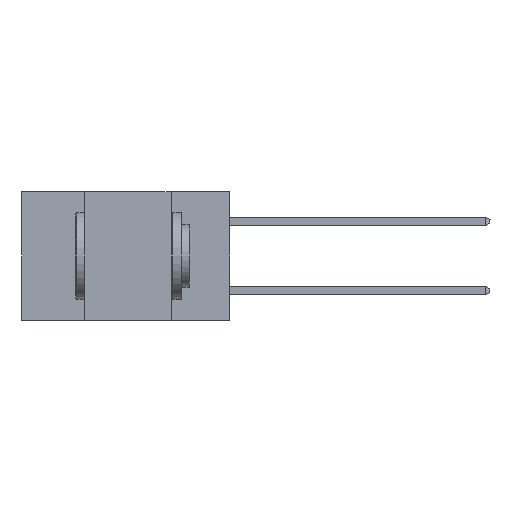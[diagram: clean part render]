
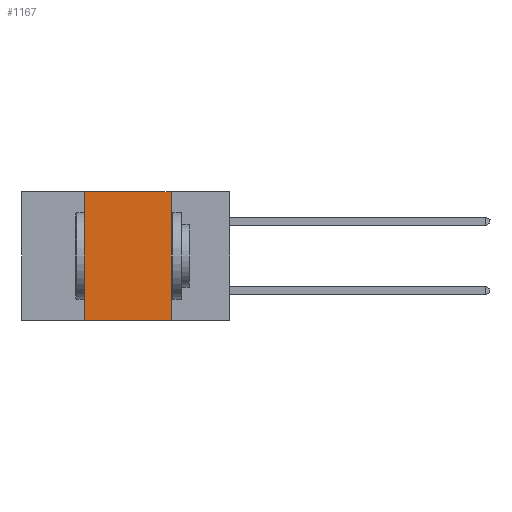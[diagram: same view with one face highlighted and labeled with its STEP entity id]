
A CAD part, left-side view. The second image highlights one B-rep face of the part: STEP entity #1167.
In plain terms, the highlighted planar face has unit normal (-1, 0, 0).
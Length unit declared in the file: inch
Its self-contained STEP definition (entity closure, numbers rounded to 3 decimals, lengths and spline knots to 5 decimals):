
#509 = CARTESIAN_POINT ( 'NONE',  ( 0., 0.6, 0. ) ) ;
#540 = ORIENTED_EDGE ( 'NONE', *, *, #13798, .F. ) ;
#863 = DIRECTION ( 'NONE',  ( 0., 0., -1. ) ) ;
#1167 = ADVANCED_FACE ( 'NONE', ( #6495 ), #5584, .F. ) ;
#1600 = ORIENTED_EDGE ( 'NONE', *, *, #5975, .F. ) ;
#2596 = VERTEX_POINT ( 'NONE', #13351 ) ;
#2643 = DIRECTION ( 'NONE',  ( 0., 0., 1. ) ) ;
#2665 = LINE ( 'NONE', #8048, #14889 ) ;
#3530 = VERTEX_POINT ( 'NONE', #11727 ) ;
#4096 = CARTESIAN_POINT ( 'NONE',  ( 0., 0.6, -0.37 ) ) ;
#4434 = LINE ( 'NONE', #4096, #7961 ) ;
#4602 = DIRECTION ( 'NONE',  ( 0., 0., -1. ) ) ;
#5203 = DIRECTION ( 'NONE',  ( 0., -1., 0. ) ) ;
#5584 = PLANE ( 'NONE',  #13331 ) ;
#5975 = EDGE_CURVE ( 'NONE', #8008, #9208, #10800, .T. ) ;
#6255 = EDGE_CURVE ( 'NONE', #2596, #8008, #15055, .T. ) ;
#6495 = FACE_OUTER_BOUND ( 'NONE', #9733, .T. ) ;
#7597 = ORIENTED_EDGE ( 'NONE', *, *, #8961, .T. ) ;
#7747 = DIRECTION ( 'NONE',  ( 0., -1., 0. ) ) ;
#7961 = VECTOR ( 'NONE', #7747, 39.37008 ) ;
#7975 = CARTESIAN_POINT ( 'NONE',  ( 0., 0.6, 0. ) ) ;
#8008 = VERTEX_POINT ( 'NONE', #11264 ) ;
#8048 = CARTESIAN_POINT ( 'NONE',  ( 0., 0.17, 0. ) ) ;
#8415 = VECTOR ( 'NONE', #5203, 39.37008 ) ;
#8571 = CARTESIAN_POINT ( 'NONE',  ( 0., 0.42, 0. ) ) ;
#8961 = EDGE_CURVE ( 'NONE', #2596, #3530, #4434, .T. ) ;
#9208 = VERTEX_POINT ( 'NONE', #15051 ) ;
#9720 = ORIENTED_EDGE ( 'NONE', *, *, #6255, .F. ) ;
#9733 = EDGE_LOOP ( 'NONE', ( #540, #1600, #9720, #7597 ) ) ;
#10800 = LINE ( 'NONE', #509, #8415 ) ;
#11264 = CARTESIAN_POINT ( 'NONE',  ( 0., 0.42, 0. ) ) ;
#11727 = CARTESIAN_POINT ( 'NONE',  ( 0., 0.17, -0.37 ) ) ;
#12666 = VECTOR ( 'NONE', #2643, 39.37008 ) ;
#13331 = AXIS2_PLACEMENT_3D ( 'NONE', #7975, #15017, #863 ) ;
#13351 = CARTESIAN_POINT ( 'NONE',  ( 0., 0.42, -0.37 ) ) ;
#13798 = EDGE_CURVE ( 'NONE', #9208, #3530, #2665, .T. ) ;
#14889 = VECTOR ( 'NONE', #4602, 39.37008 ) ;
#15017 = DIRECTION ( 'NONE',  ( 1., 0., 0. ) ) ;
#15051 = CARTESIAN_POINT ( 'NONE',  ( 0., 0.17, 0. ) ) ;
#15055 = LINE ( 'NONE', #8571, #12666 ) ;
